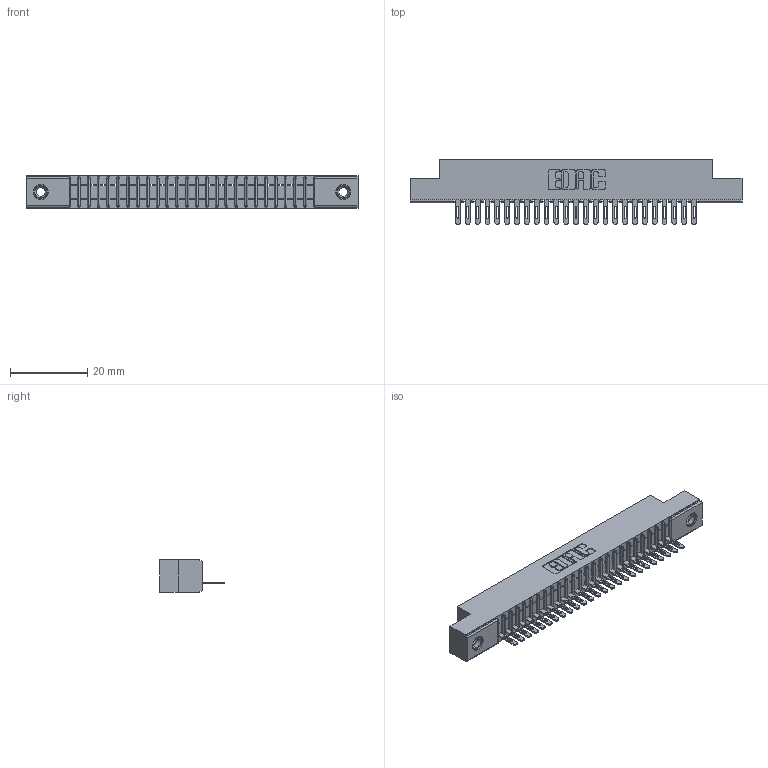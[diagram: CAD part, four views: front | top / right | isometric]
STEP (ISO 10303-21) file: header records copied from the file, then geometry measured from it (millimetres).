
FILE_DESCRIPTION (( 'STEP AP203' ), '1' );
FILE_NAME ('341-025-500-108.STEP', '2018-08-06T18:17:50', ( '' ), ( '' ), 'SwSTEP 2.0', 'SolidWorks 2016', '' );
FILE_SCHEMA (( 'CONFIG_CONTROL_DESIGN' ));
Length unit declared in the file: inch
Products named in the file (4): 341 Part_.156 (3.96) Dia Mounting Holes; 341-292-001_341-292-100; 345-250-001_345-250-003-102; 341-025-500-108
Assembly tree (28 placements, depth 2):
  341-025-500-108
    341 Part_.156 (3.96) Dia Mounting Holes
    341-292-001_341-292-100  x25
    345-250-001_345-250-003-102  x2
Bounding box: 85.72 x 16.69 x 8.38 mm (x, y, z)
Volume: 4719.1 mm3; surface area: 9042.8 mm2
Topology: 28 solids, 28 shells, 2226 faces, 6377 edges, 4090 vertices
Faces by surface type: plane 1325, cylinder 785, sphere 52, torus 52, cone 12
Entity records: 32913 total; most frequent: CARTESIAN_POINT 5561, ORIENTED_EDGE 5542, DIRECTION 5397, EDGE_CURVE 2771, LINE 2213, VECTOR 2213, VERTEX_POINT 1756, AXIS2_PLACEMENT_3D 1592
